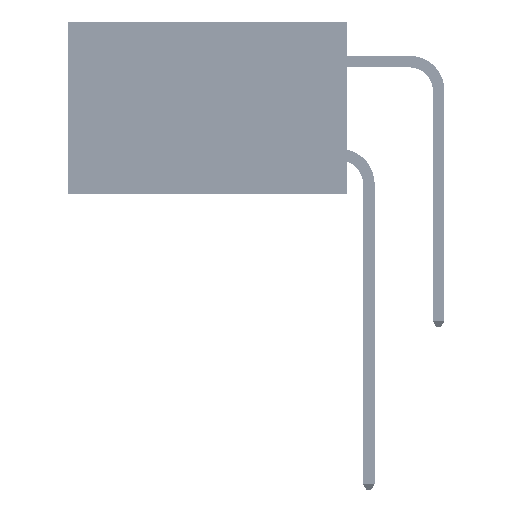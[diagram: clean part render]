
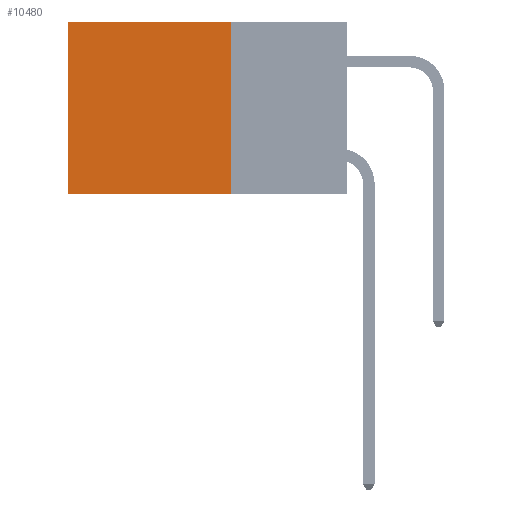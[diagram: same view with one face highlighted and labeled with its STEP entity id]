
A CAD part, left-side view. The second image highlights one B-rep face of the part: STEP entity #10480.
In plain terms, the highlighted planar face has unit normal (-1, 0, 0).
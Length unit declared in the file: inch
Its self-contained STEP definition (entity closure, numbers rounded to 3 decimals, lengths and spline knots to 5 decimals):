
#1137 = DIRECTION ( 'NONE',  ( 0., 1., 0. ) ) ;
#2719 = VERTEX_POINT ( 'NONE', #42085 ) ;
#2880 = LINE ( 'NONE', #46311, #48846 ) ;
#4322 = VECTOR ( 'NONE', #1137, 39.37008 ) ;
#6423 = LINE ( 'NONE', #40196, #38991 ) ;
#6880 = LINE ( 'NONE', #21157, #4322 ) ;
#10480 = ADVANCED_FACE ( 'NONE', ( #30029 ), #31626, .F. ) ;
#12412 = DIRECTION ( 'NONE',  ( 0., 1., 0. ) ) ;
#15231 = CARTESIAN_POINT ( 'NONE',  ( 0.2875, 0.25, 0. ) ) ;
#17053 = ORIENTED_EDGE ( 'NONE', *, *, #49132, .F. ) ;
#17765 = VECTOR ( 'NONE', #12412, 39.37008 ) ;
#18033 = EDGE_LOOP ( 'NONE', ( #28147, #17053, #46676, #32519 ) ) ;
#20760 = CARTESIAN_POINT ( 'NONE',  ( 0.2875, 0.25, -0.37 ) ) ;
#21157 = CARTESIAN_POINT ( 'NONE',  ( 0.2875, 0.25, 0. ) ) ;
#22118 = VERTEX_POINT ( 'NONE', #41383 ) ;
#23741 = EDGE_CURVE ( 'NONE', #48941, #2719, #6423, .T. ) ;
#23929 = DIRECTION ( 'NONE',  ( 0., 0., -1. ) ) ;
#27377 = CARTESIAN_POINT ( 'NONE',  ( 0.2875, 0.25, 0. ) ) ;
#28147 = ORIENTED_EDGE ( 'NONE', *, *, #50675, .T. ) ;
#30029 = FACE_OUTER_BOUND ( 'NONE', #18033, .T. ) ;
#31626 = PLANE ( 'NONE',  #42926 ) ;
#32093 = EDGE_CURVE ( 'NONE', #48941, #22118, #6880, .T. ) ;
#32519 = ORIENTED_EDGE ( 'NONE', *, *, #32093, .T. ) ;
#33653 = DIRECTION ( 'NONE',  ( 0., 0., -1. ) ) ;
#34288 = LINE ( 'NONE', #20760, #17765 ) ;
#35940 = DIRECTION ( 'NONE',  ( 1., 0., 0. ) ) ;
#38991 = VECTOR ( 'NONE', #23929, 39.37008 ) ;
#39860 = DIRECTION ( 'NONE',  ( 0., 0., -1. ) ) ;
#40196 = CARTESIAN_POINT ( 'NONE',  ( 0.2875, 0.25, 0. ) ) ;
#40430 = VERTEX_POINT ( 'NONE', #48160 ) ;
#41383 = CARTESIAN_POINT ( 'NONE',  ( 0.2875, 0.6, 0. ) ) ;
#42085 = CARTESIAN_POINT ( 'NONE',  ( 0.2875, 0.25, -0.37 ) ) ;
#42926 = AXIS2_PLACEMENT_3D ( 'NONE', #15231, #35940, #39860 ) ;
#46311 = CARTESIAN_POINT ( 'NONE',  ( 0.2875, 0.6, 0. ) ) ;
#46676 = ORIENTED_EDGE ( 'NONE', *, *, #23741, .F. ) ;
#48160 = CARTESIAN_POINT ( 'NONE',  ( 0.2875, 0.6, -0.37 ) ) ;
#48846 = VECTOR ( 'NONE', #33653, 39.37008 ) ;
#48941 = VERTEX_POINT ( 'NONE', #27377 ) ;
#49132 = EDGE_CURVE ( 'NONE', #2719, #40430, #34288, .T. ) ;
#50675 = EDGE_CURVE ( 'NONE', #22118, #40430, #2880, .T. ) ;
